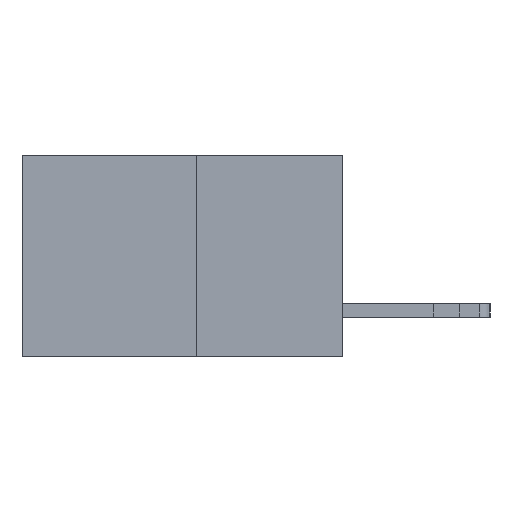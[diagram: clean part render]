
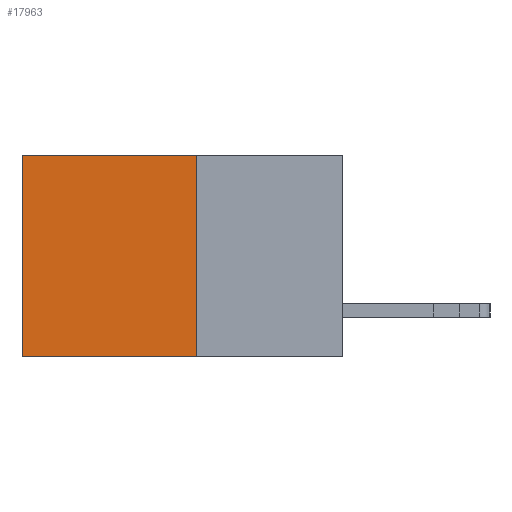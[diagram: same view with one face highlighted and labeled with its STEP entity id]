
A CAD part, left-side view. The second image highlights one B-rep face of the part: STEP entity #17963.
In plain terms, the highlighted planar face has unit normal (-1, 0, 0).
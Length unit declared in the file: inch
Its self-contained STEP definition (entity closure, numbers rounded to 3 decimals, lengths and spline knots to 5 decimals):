
#14 = VECTOR ( 'NONE', #3968, 39.37008 ) ;
#1141 = AXIS2_PLACEMENT_3D ( 'NONE', #19312, #6254, #21506 ) ;
#1306 = EDGE_LOOP ( 'NONE', ( #3744, #11228, #22627, #14099 ) ) ;
#1755 = CARTESIAN_POINT ( 'NONE',  ( 0.277, 0.27, -0.37 ) ) ;
#2770 = LINE ( 'NONE', #27429, #8658 ) ;
#3635 = VERTEX_POINT ( 'NONE', #27295 ) ;
#3707 = CARTESIAN_POINT ( 'NONE',  ( 0.277, 0.59, -0.37 ) ) ;
#3744 = ORIENTED_EDGE ( 'NONE', *, *, #21287, .T. ) ;
#3968 = DIRECTION ( 'NONE',  ( 0., 1., 0. ) ) ;
#4037 = CARTESIAN_POINT ( 'NONE',  ( 0.277, 0.27, -0.37 ) ) ;
#4928 = LINE ( 'NONE', #24059, #20993 ) ;
#6254 = DIRECTION ( 'NONE',  ( 1., 0., 0. ) ) ;
#6854 = FACE_OUTER_BOUND ( 'NONE', #1306, .T. ) ;
#8658 = VECTOR ( 'NONE', #10172, 39.37008 ) ;
#10172 = DIRECTION ( 'NONE',  ( 0., 1., 0. ) ) ;
#11228 = ORIENTED_EDGE ( 'NONE', *, *, #25265, .F. ) ;
#12845 = EDGE_CURVE ( 'NONE', #25637, #3635, #17437, .T. ) ;
#14099 = ORIENTED_EDGE ( 'NONE', *, *, #17228, .T. ) ;
#16938 = PLANE ( 'NONE',  #1141 ) ;
#17228 = EDGE_CURVE ( 'NONE', #25637, #22036, #2770, .T. ) ;
#17279 = VERTEX_POINT ( 'NONE', #3707 ) ;
#17437 = LINE ( 'NONE', #4037, #19485 ) ;
#17444 = LINE ( 'NONE', #1755, #14 ) ;
#17963 = ADVANCED_FACE ( 'NONE', ( #6854 ), #16938, .F. ) ;
#19312 = CARTESIAN_POINT ( 'NONE',  ( 0.277, 0.27, -0.37 ) ) ;
#19485 = VECTOR ( 'NONE', #21487, 39.37008 ) ;
#20993 = VECTOR ( 'NONE', #26190, 39.37008 ) ;
#21287 = EDGE_CURVE ( 'NONE', #22036, #17279, #4928, .T. ) ;
#21487 = DIRECTION ( 'NONE',  ( 0., 0., -1. ) ) ;
#21506 = DIRECTION ( 'NONE',  ( 0., 0., -1. ) ) ;
#22036 = VERTEX_POINT ( 'NONE', #26626 ) ;
#22627 = ORIENTED_EDGE ( 'NONE', *, *, #12845, .F. ) ;
#24059 = CARTESIAN_POINT ( 'NONE',  ( 0.277, 0.59, -0.37 ) ) ;
#24806 = CARTESIAN_POINT ( 'NONE',  ( 0.277, 0.27, 0. ) ) ;
#25265 = EDGE_CURVE ( 'NONE', #3635, #17279, #17444, .T. ) ;
#25637 = VERTEX_POINT ( 'NONE', #24806 ) ;
#26190 = DIRECTION ( 'NONE',  ( 0., 0., -1. ) ) ;
#26626 = CARTESIAN_POINT ( 'NONE',  ( 0.277, 0.59, 0. ) ) ;
#27295 = CARTESIAN_POINT ( 'NONE',  ( 0.277, 0.27, -0.37 ) ) ;
#27429 = CARTESIAN_POINT ( 'NONE',  ( 0.277, 0.27, 0. ) ) ;
